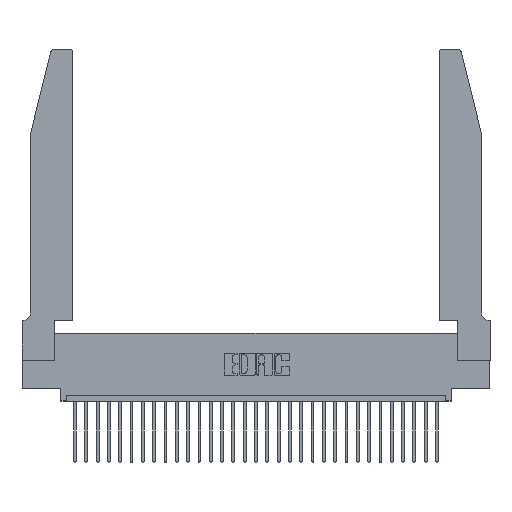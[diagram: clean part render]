
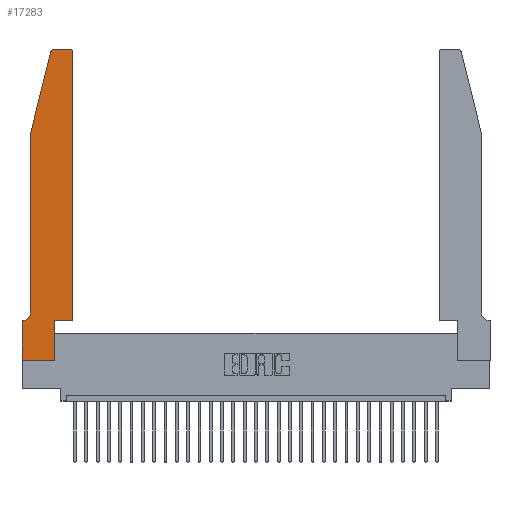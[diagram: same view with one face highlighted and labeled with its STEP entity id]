
A CAD part, top view. The second image highlights one B-rep face of the part: STEP entity #17283.
In plain terms, the highlighted planar face has unit normal (0, 0, 1).
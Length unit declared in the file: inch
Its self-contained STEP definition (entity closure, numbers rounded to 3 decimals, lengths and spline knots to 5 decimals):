
#662 = CARTESIAN_POINT ( 'NONE',  ( 0.4205, 2.75, 0.37 ) ) ;
#831 = DIRECTION ( 'NONE',  ( 0., -1., 0. ) ) ;
#833 = DIRECTION ( 'NONE',  ( -1., 0., 0. ) ) ;
#964 = VECTOR ( 'NONE', #7103, 39.37008 ) ;
#1141 = VERTEX_POINT ( 'NONE', #26756 ) ;
#1388 = ORIENTED_EDGE ( 'NONE', *, *, #24060, .T. ) ;
#1771 = ORIENTED_EDGE ( 'NONE', *, *, #12461, .T. ) ;
#1947 = LINE ( 'NONE', #17235, #28867 ) ;
#2032 = VERTEX_POINT ( 'NONE', #27942 ) ;
#2161 = EDGE_CURVE ( 'NONE', #27021, #8853, #1947, .T. ) ;
#2250 = VECTOR ( 'NONE', #831, 39.37008 ) ;
#3124 = VECTOR ( 'NONE', #10422, 39.37008 ) ;
#3926 = LINE ( 'NONE', #12253, #23005 ) ;
#4322 = EDGE_CURVE ( 'NONE', #1141, #29682, #25020, .T. ) ;
#4459 = DIRECTION ( 'NONE',  ( 0., 0., 1. ) ) ;
#4613 = CARTESIAN_POINT ( 'NONE',  ( 0.0755, 2., 0.37 ) ) ;
#5179 = ORIENTED_EDGE ( 'NONE', *, *, #19364, .T. ) ;
#5630 = CARTESIAN_POINT ( 'NONE',  ( 0., 0., 0.37 ) ) ;
#6020 = LINE ( 'NONE', #13797, #6754 ) ;
#6408 = CIRCLE ( 'NONE', #15674, 0.03 ) ;
#6754 = VECTOR ( 'NONE', #9062, 39.37008 ) ;
#7103 = DIRECTION ( 'NONE',  ( 0., 1., 0. ) ) ;
#7416 = VERTEX_POINT ( 'NONE', #14194 ) ;
#8053 = CARTESIAN_POINT ( 'NONE',  ( 0.284, 2.75, 0.37 ) ) ;
#8853 = VERTEX_POINT ( 'NONE', #4613 ) ;
#8901 = CIRCLE ( 'NONE', #20174, 0.07 ) ;
#8942 = LINE ( 'NONE', #24173, #2250 ) ;
#9062 = DIRECTION ( 'NONE',  ( -1., 0., 0. ) ) ;
#9106 = EDGE_CURVE ( 'NONE', #14866, #1141, #3926, .T. ) ;
#9229 = CARTESIAN_POINT ( 'NONE',  ( 0.4205, 2.72, 0.37 ) ) ;
#9892 = VERTEX_POINT ( 'NONE', #26687 ) ;
#10006 = VERTEX_POINT ( 'NONE', #8053 ) ;
#10422 = DIRECTION ( 'NONE',  ( 0., -1., 0. ) ) ;
#10516 = LINE ( 'NONE', #17203, #21030 ) ;
#10548 = CARTESIAN_POINT ( 'NONE',  ( 0.2605, 2.75, 0.37 ) ) ;
#10703 = EDGE_CURVE ( 'NONE', #27199, #9892, #23710, .T. ) ;
#10858 = ORIENTED_EDGE ( 'NONE', *, *, #17365, .T. ) ;
#10988 = ORIENTED_EDGE ( 'NONE', *, *, #22063, .T. ) ;
#11523 = VECTOR ( 'NONE', #29611, 39.37008 ) ;
#11623 = DIRECTION ( 'NONE',  ( 1., 0., 0. ) ) ;
#12253 = CARTESIAN_POINT ( 'NONE',  ( 0.4505, 0.35, 0.37 ) ) ;
#12440 = CARTESIAN_POINT ( 'NONE',  ( 0., 0.35, 0.37 ) ) ;
#12461 = EDGE_CURVE ( 'NONE', #24058, #10006, #19078, .T. ) ;
#12897 = CARTESIAN_POINT ( 'NONE',  ( 0.4505, 0.35, 0.37 ) ) ;
#13056 = VECTOR ( 'NONE', #833, 39.37008 ) ;
#13797 = CARTESIAN_POINT ( 'NONE',  ( 0.0755, 0.35, 0.37 ) ) ;
#14194 = CARTESIAN_POINT ( 'NONE',  ( 0.0055, 0.35, 0.37 ) ) ;
#14744 = ORIENTED_EDGE ( 'NONE', *, *, #10703, .T. ) ;
#14866 = VERTEX_POINT ( 'NONE', #25707 ) ;
#15146 = DIRECTION ( 'NONE',  ( -0.239, -0.971, 0. ) ) ;
#15237 = ORIENTED_EDGE ( 'NONE', *, *, #18283, .T. ) ;
#15674 = AXIS2_PLACEMENT_3D ( 'NONE', #9229, #25958, #11623 ) ;
#16210 = AXIS2_PLACEMENT_3D ( 'NONE', #30706, #28501, #26004 ) ;
#17038 = ORIENTED_EDGE ( 'NONE', *, *, #9106, .T. ) ;
#17203 = CARTESIAN_POINT ( 'NONE',  ( 0., 0., 0.37 ) ) ;
#17235 = CARTESIAN_POINT ( 'NONE',  ( 0.0755, 2., 0.37 ) ) ;
#17283 = ADVANCED_FACE ( 'NONE', ( #26919 ), #26175, .T. ) ;
#17365 = EDGE_CURVE ( 'NONE', #8853, #2032, #8942, .T. ) ;
#17444 = DIRECTION ( 'NONE',  ( -1., 0., 0. ) ) ;
#17643 = CARTESIAN_POINT ( 'NONE',  ( 0.0055, 0.42, 0.37 ) ) ;
#17830 = LINE ( 'NONE', #21568, #964 ) ;
#18283 = EDGE_CURVE ( 'NONE', #10006, #27021, #28339, .T. ) ;
#18912 = DIRECTION ( 'NONE',  ( 1., 0., 0. ) ) ;
#19078 = LINE ( 'NONE', #10548, #13056 ) ;
#19364 = EDGE_CURVE ( 'NONE', #30665, #14866, #17830, .T. ) ;
#19581 = AXIS2_PLACEMENT_3D ( 'NONE', #25856, #4459, #18912 ) ;
#19589 = DIRECTION ( 'NONE',  ( 1., 0., 0. ) ) ;
#20174 = AXIS2_PLACEMENT_3D ( 'NONE', #17643, #24728, #17444 ) ;
#21030 = VECTOR ( 'NONE', #19589, 39.37008 ) ;
#21568 = CARTESIAN_POINT ( 'NONE',  ( 0.2865, 0.35, 0.37 ) ) ;
#21700 = EDGE_CURVE ( 'NONE', #29682, #24058, #6408, .T. ) ;
#22063 = EDGE_CURVE ( 'NONE', #7416, #27199, #6020, .T. ) ;
#22989 = ORIENTED_EDGE ( 'NONE', *, *, #2161, .T. ) ;
#23005 = VECTOR ( 'NONE', #28675, 39.37008 ) ;
#23710 = LINE ( 'NONE', #5630, #3124 ) ;
#24058 = VERTEX_POINT ( 'NONE', #662 ) ;
#24060 = EDGE_CURVE ( 'NONE', #2032, #7416, #8901, .T. ) ;
#24173 = CARTESIAN_POINT ( 'NONE',  ( 0.0755, 2., 0.37 ) ) ;
#24489 = ORIENTED_EDGE ( 'NONE', *, *, #4322, .T. ) ;
#24728 = DIRECTION ( 'NONE',  ( 0., 0., -1. ) ) ;
#24950 = CARTESIAN_POINT ( 'NONE',  ( 0.4505, 2.72, 0.37 ) ) ;
#25020 = LINE ( 'NONE', #12897, #11523 ) ;
#25234 = CARTESIAN_POINT ( 'NONE',  ( 0.2865, 0., 0.37 ) ) ;
#25707 = CARTESIAN_POINT ( 'NONE',  ( 0.2865, 0.35, 0.37 ) ) ;
#25718 = EDGE_LOOP ( 'NONE', ( #1771, #15237, #22989, #10858, #1388, #10988, #14744, #28394, #5179, #17038, #24489, #30752 ) ) ;
#25856 = CARTESIAN_POINT ( 'NONE',  ( 0., 0.35, 0.37 ) ) ;
#25958 = DIRECTION ( 'NONE',  ( 0., 0., 1. ) ) ;
#26004 = DIRECTION ( 'NONE',  ( 1., 0., 0. ) ) ;
#26175 = PLANE ( 'NONE',  #19581 ) ;
#26236 = CARTESIAN_POINT ( 'NONE',  ( 0.25487, 2.72718, 0.37 ) ) ;
#26687 = CARTESIAN_POINT ( 'NONE',  ( 0., 0., 0.37 ) ) ;
#26756 = CARTESIAN_POINT ( 'NONE',  ( 0.4505, 0.35, 0.37 ) ) ;
#26919 = FACE_OUTER_BOUND ( 'NONE', #25718, .T. ) ;
#27021 = VERTEX_POINT ( 'NONE', #26236 ) ;
#27199 = VERTEX_POINT ( 'NONE', #12440 ) ;
#27942 = CARTESIAN_POINT ( 'NONE',  ( 0.0755, 0.42, 0.37 ) ) ;
#28339 = CIRCLE ( 'NONE', #16210, 0.03 ) ;
#28394 = ORIENTED_EDGE ( 'NONE', *, *, #28975, .T. ) ;
#28501 = DIRECTION ( 'NONE',  ( 0., 0., 1. ) ) ;
#28675 = DIRECTION ( 'NONE',  ( 1., 0., 0. ) ) ;
#28867 = VECTOR ( 'NONE', #15146, 39.37008 ) ;
#28975 = EDGE_CURVE ( 'NONE', #9892, #30665, #10516, .T. ) ;
#29611 = DIRECTION ( 'NONE',  ( 0., 1., 0. ) ) ;
#29682 = VERTEX_POINT ( 'NONE', #24950 ) ;
#30665 = VERTEX_POINT ( 'NONE', #25234 ) ;
#30706 = CARTESIAN_POINT ( 'NONE',  ( 0.284, 2.72, 0.37 ) ) ;
#30752 = ORIENTED_EDGE ( 'NONE', *, *, #21700, .T. ) ;
